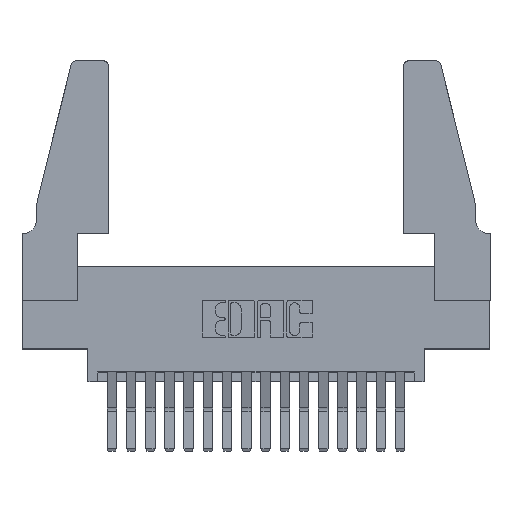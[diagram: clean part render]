
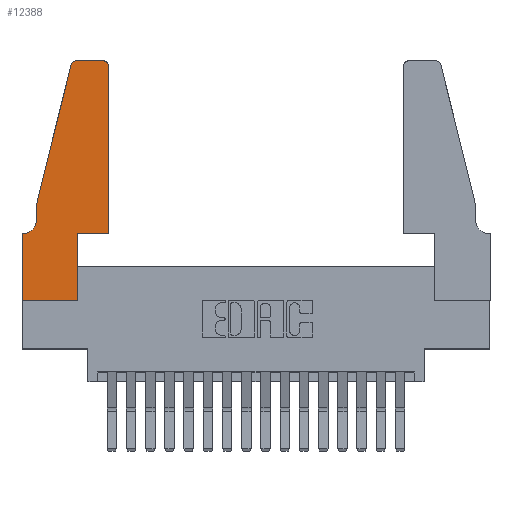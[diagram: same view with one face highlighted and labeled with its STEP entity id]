
A CAD part, top view. The second image highlights one B-rep face of the part: STEP entity #12388.
In plain terms, the highlighted planar face has unit normal (0, 0, 1).
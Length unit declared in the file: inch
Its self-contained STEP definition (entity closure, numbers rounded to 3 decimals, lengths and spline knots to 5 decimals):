
#32 = EDGE_CURVE ( 'NONE', #18162, #10672, #15482, .T. ) ;
#37 = CARTESIAN_POINT ( 'NONE',  ( 0., 0.35, 0.37 ) ) ;
#157 = VECTOR ( 'NONE', #1128, 39.37008 ) ;
#204 = DIRECTION ( 'NONE',  ( 0., -1., 0. ) ) ;
#571 = FACE_OUTER_BOUND ( 'NONE', #18451, .T. ) ;
#614 = LINE ( 'NONE', #4781, #15410 ) ;
#754 = CARTESIAN_POINT ( 'NONE',  ( 0.25487, 1.22718, 0.37 ) ) ;
#879 = CIRCLE ( 'NONE', #18454, 0.03 ) ;
#884 = ORIENTED_EDGE ( 'NONE', *, *, #32, .T. ) ;
#1064 = LINE ( 'NONE', #14365, #13327 ) ;
#1128 = DIRECTION ( 'NONE',  ( 0., -1., 0. ) ) ;
#1190 = VERTEX_POINT ( 'NONE', #18142 ) ;
#1343 = VERTEX_POINT ( 'NONE', #1495 ) ;
#1381 = DIRECTION ( 'NONE',  ( 1., 0., 0. ) ) ;
#1442 = ORIENTED_EDGE ( 'NONE', *, *, #15287, .T. ) ;
#1495 = CARTESIAN_POINT ( 'NONE',  ( 0.2865, 0.35, 0.37 ) ) ;
#1621 = AXIS2_PLACEMENT_3D ( 'NONE', #7249, #12688, #10076 ) ;
#1760 = DIRECTION ( 'NONE',  ( -1., 0., 0. ) ) ;
#1800 = LINE ( 'NONE', #12284, #8563 ) ;
#1817 = EDGE_CURVE ( 'NONE', #15446, #3032, #16962, .T. ) ;
#1998 = CARTESIAN_POINT ( 'NONE',  ( 0.2865, 0., 0.37 ) ) ;
#2036 = DIRECTION ( 'NONE',  ( 0., 0., 1. ) ) ;
#2741 = EDGE_CURVE ( 'NONE', #15458, #10921, #1064, .T. ) ;
#2889 = CARTESIAN_POINT ( 'NONE',  ( 0.4205, 1.25, 0.37 ) ) ;
#2974 = VECTOR ( 'NONE', #13360, 39.37008 ) ;
#3013 = VECTOR ( 'NONE', #1381, 39.37008 ) ;
#3032 = VERTEX_POINT ( 'NONE', #754 ) ;
#3306 = DIRECTION ( 'NONE',  ( 0., 0., 1. ) ) ;
#4052 = CARTESIAN_POINT ( 'NONE',  ( 0., 0.35, 0.37 ) ) ;
#4303 = ORIENTED_EDGE ( 'NONE', *, *, #8326, .T. ) ;
#4726 = ORIENTED_EDGE ( 'NONE', *, *, #2741, .T. ) ;
#4781 = CARTESIAN_POINT ( 'NONE',  ( 0.2865, 0.35, 0.37 ) ) ;
#5013 = CARTESIAN_POINT ( 'NONE',  ( 0.0755, 0.5, 0.37 ) ) ;
#5106 = DIRECTION ( 'NONE',  ( 0., 1., 0. ) ) ;
#5367 = CARTESIAN_POINT ( 'NONE',  ( 0.284, 1.25, 0.37 ) ) ;
#5916 = CARTESIAN_POINT ( 'NONE',  ( 0.0755, 0.5, 0.37 ) ) ;
#6254 = VECTOR ( 'NONE', #14830, 39.37008 ) ;
#6402 = CARTESIAN_POINT ( 'NONE',  ( 0., 0., 0.37 ) ) ;
#6411 = CARTESIAN_POINT ( 'NONE',  ( 0.4505, 1.22, 0.37 ) ) ;
#6601 = ORIENTED_EDGE ( 'NONE', *, *, #15947, .T. ) ;
#7249 = CARTESIAN_POINT ( 'NONE',  ( 0.0055, 0.42, 0.37 ) ) ;
#7362 = CARTESIAN_POINT ( 'NONE',  ( 0.0755, 0.5, 0.37 ) ) ;
#7752 = CARTESIAN_POINT ( 'NONE',  ( 0.0755, 0.35, 0.37 ) ) ;
#8306 = ORIENTED_EDGE ( 'NONE', *, *, #13349, .T. ) ;
#8326 = EDGE_CURVE ( 'NONE', #1343, #15458, #9717, .T. ) ;
#8517 = ORIENTED_EDGE ( 'NONE', *, *, #17769, .T. ) ;
#8563 = VECTOR ( 'NONE', #15222, 39.37008 ) ;
#8837 = VERTEX_POINT ( 'NONE', #2889 ) ;
#9028 = CARTESIAN_POINT ( 'NONE',  ( 0.0755, 0.42, 0.37 ) ) ;
#9036 = VERTEX_POINT ( 'NONE', #5916 ) ;
#9103 = ORIENTED_EDGE ( 'NONE', *, *, #1817, .T. ) ;
#9717 = LINE ( 'NONE', #9942, #3013 ) ;
#9737 = DIRECTION ( 'NONE',  ( 0., 0., 1. ) ) ;
#9942 = CARTESIAN_POINT ( 'NONE',  ( 0.4505, 0.35, 0.37 ) ) ;
#10002 = LINE ( 'NONE', #7362, #12238 ) ;
#10076 = DIRECTION ( 'NONE',  ( -1., 0., 0. ) ) ;
#10335 = DIRECTION ( 'NONE',  ( 1., 0., 0. ) ) ;
#10672 = VERTEX_POINT ( 'NONE', #37 ) ;
#10921 = VERTEX_POINT ( 'NONE', #6411 ) ;
#11214 = EDGE_CURVE ( 'NONE', #10672, #1190, #11792, .T. ) ;
#11792 = LINE ( 'NONE', #6402, #157 ) ;
#12238 = VECTOR ( 'NONE', #204, 39.37008 ) ;
#12284 = CARTESIAN_POINT ( 'NONE',  ( 0., 0., 0.37 ) ) ;
#12388 = ADVANCED_FACE ( 'NONE', ( #571 ), #13824, .T. ) ;
#12635 = ORIENTED_EDGE ( 'NONE', *, *, #11214, .T. ) ;
#12688 = DIRECTION ( 'NONE',  ( 0., 0., -1. ) ) ;
#13326 = VECTOR ( 'NONE', #1760, 39.37008 ) ;
#13327 = VECTOR ( 'NONE', #14253, 39.37008 ) ;
#13349 = EDGE_CURVE ( 'NONE', #1190, #18085, #1800, .T. ) ;
#13360 = DIRECTION ( 'NONE',  ( -1., 0., 0. ) ) ;
#13427 = AXIS2_PLACEMENT_3D ( 'NONE', #4052, #2036, #13480 ) ;
#13480 = DIRECTION ( 'NONE',  ( 1., 0., 0. ) ) ;
#13824 = PLANE ( 'NONE',  #13427 ) ;
#13825 = CARTESIAN_POINT ( 'NONE',  ( 0.4505, 0.35, 0.37 ) ) ;
#14002 = CARTESIAN_POINT ( 'NONE',  ( 0.284, 1.22, 0.37 ) ) ;
#14253 = DIRECTION ( 'NONE',  ( 0., 1., 0. ) ) ;
#14365 = CARTESIAN_POINT ( 'NONE',  ( 0.4505, 0.35, 0.37 ) ) ;
#14752 = CARTESIAN_POINT ( 'NONE',  ( 0.2605, 1.25, 0.37 ) ) ;
#14773 = CARTESIAN_POINT ( 'NONE',  ( 0.4205, 1.22, 0.37 ) ) ;
#14830 = DIRECTION ( 'NONE',  ( -0.239, -0.971, 0. ) ) ;
#14877 = LINE ( 'NONE', #14752, #13326 ) ;
#15109 = AXIS2_PLACEMENT_3D ( 'NONE', #14002, #9737, #16832 ) ;
#15222 = DIRECTION ( 'NONE',  ( 1., 0., 0. ) ) ;
#15287 = EDGE_CURVE ( 'NONE', #10921, #8837, #879, .T. ) ;
#15315 = CIRCLE ( 'NONE', #1621, 0.07 ) ;
#15410 = VECTOR ( 'NONE', #5106, 39.37008 ) ;
#15446 = VERTEX_POINT ( 'NONE', #5367 ) ;
#15458 = VERTEX_POINT ( 'NONE', #13825 ) ;
#15482 = LINE ( 'NONE', #7752, #2974 ) ;
#15614 = EDGE_CURVE ( 'NONE', #3032, #9036, #17826, .T. ) ;
#15947 = EDGE_CURVE ( 'NONE', #18085, #1343, #614, .T. ) ;
#16462 = EDGE_CURVE ( 'NONE', #9036, #16926, #10002, .T. ) ;
#16486 = EDGE_CURVE ( 'NONE', #8837, #15446, #14877, .T. ) ;
#16832 = DIRECTION ( 'NONE',  ( 1., 0., 0. ) ) ;
#16833 = ORIENTED_EDGE ( 'NONE', *, *, #15614, .T. ) ;
#16926 = VERTEX_POINT ( 'NONE', #9028 ) ;
#16962 = CIRCLE ( 'NONE', #15109, 0.03 ) ;
#17009 = CARTESIAN_POINT ( 'NONE',  ( 0.0055, 0.35, 0.37 ) ) ;
#17626 = ORIENTED_EDGE ( 'NONE', *, *, #16486, .T. ) ;
#17769 = EDGE_CURVE ( 'NONE', #16926, #18162, #15315, .T. ) ;
#17826 = LINE ( 'NONE', #5013, #6254 ) ;
#18085 = VERTEX_POINT ( 'NONE', #1998 ) ;
#18142 = CARTESIAN_POINT ( 'NONE',  ( 0., 0., 0.37 ) ) ;
#18162 = VERTEX_POINT ( 'NONE', #17009 ) ;
#18219 = ORIENTED_EDGE ( 'NONE', *, *, #16462, .T. ) ;
#18451 = EDGE_LOOP ( 'NONE', ( #17626, #9103, #16833, #18219, #8517, #884, #12635, #8306, #6601, #4303, #4726, #1442 ) ) ;
#18454 = AXIS2_PLACEMENT_3D ( 'NONE', #14773, #3306, #10335 ) ;
